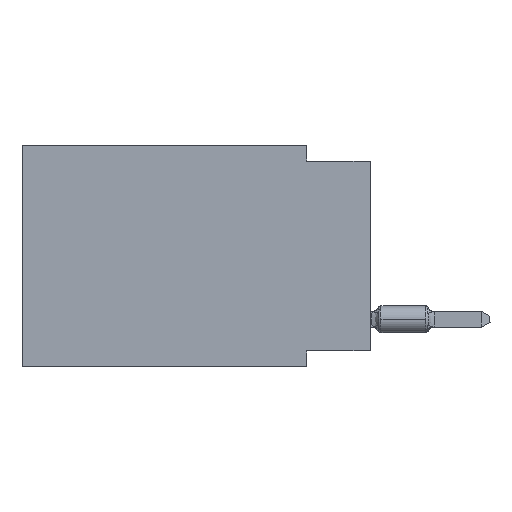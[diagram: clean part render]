
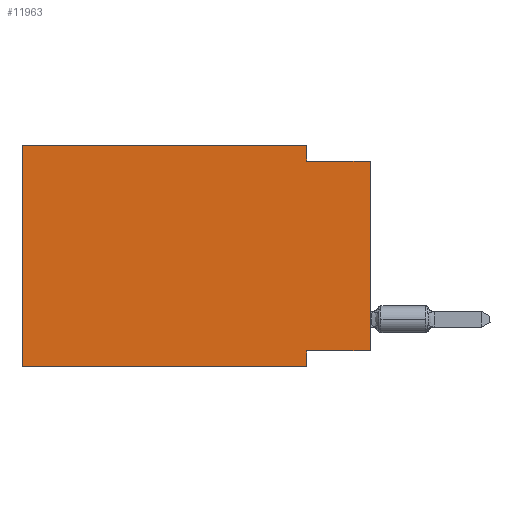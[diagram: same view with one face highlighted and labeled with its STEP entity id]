
A CAD part, left-side view. The second image highlights one B-rep face of the part: STEP entity #11963.
In plain terms, the highlighted planar face has unit normal (-1, 0, 0).
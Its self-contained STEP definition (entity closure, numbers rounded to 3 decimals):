
#720 = VERTEX_POINT ( 'NONE', #41587 ) ;
#2202 = DIRECTION ( 'NONE',  ( 1., 0., 0. ) ) ;
#2887 = ORIENTED_EDGE ( 'NONE', *, *, #34337, .F. ) ;
#4455 = EDGE_CURVE ( 'NONE', #20616, #720, #30341, .T. ) ;
#5521 = VECTOR ( 'NONE', #42073, 1000. ) ;
#6248 = VERTEX_POINT ( 'NONE', #16969 ) ;
#6534 = ORIENTED_EDGE ( 'NONE', *, *, #30725, .F. ) ;
#6631 = VECTOR ( 'NONE', #8242, 1000. ) ;
#7049 = LINE ( 'NONE', #21223, #22785 ) ;
#7694 = EDGE_LOOP ( 'NONE', ( #36475, #6534, #2887, #10210, #45464, #29347, #35352, #25045 ) ) ;
#7738 = CARTESIAN_POINT ( 'NONE',  ( 0., 0., -8.255 ) ) ;
#8242 = DIRECTION ( 'NONE',  ( 0., -1., 0. ) ) ;
#8976 = CARTESIAN_POINT ( 'NONE',  ( 0., 13.97, 0. ) ) ;
#10210 = ORIENTED_EDGE ( 'NONE', *, *, #4455, .F. ) ;
#10689 = VERTEX_POINT ( 'NONE', #41437 ) ;
#11297 = CARTESIAN_POINT ( 'NONE',  ( 0., 0., -0.635 ) ) ;
#11431 = DIRECTION ( 'NONE',  ( 0., 0., 1. ) ) ;
#11503 = LINE ( 'NONE', #19587, #6631 ) ;
#11963 = ADVANCED_FACE ( 'NONE', ( #30326 ), #44464, .F. ) ;
#12104 = CARTESIAN_POINT ( 'NONE',  ( 0., 2.54, -8.89 ) ) ;
#12562 = DIRECTION ( 'NONE',  ( 0., 0., -1. ) ) ;
#13412 = VECTOR ( 'NONE', #33971, 1000. ) ;
#13740 = VECTOR ( 'NONE', #12562, 1000. ) ;
#13763 = LINE ( 'NONE', #41613, #5521 ) ;
#15521 = VECTOR ( 'NONE', #20331, 1000. ) ;
#15610 = CARTESIAN_POINT ( 'NONE',  ( 0., 0., 0. ) ) ;
#15676 = EDGE_CURVE ( 'NONE', #17171, #20616, #43720, .T. ) ;
#16839 = CARTESIAN_POINT ( 'NONE',  ( 0., 13.97, 0. ) ) ;
#16969 = CARTESIAN_POINT ( 'NONE',  ( 0., 2.54, -8.89 ) ) ;
#17171 = VERTEX_POINT ( 'NONE', #43121 ) ;
#17316 = CARTESIAN_POINT ( 'NONE',  ( 0., 2.54, -0.635 ) ) ;
#19587 = CARTESIAN_POINT ( 'NONE',  ( 0., 13.97, -8.89 ) ) ;
#19666 = CARTESIAN_POINT ( 'NONE',  ( 0., 0., -8.255 ) ) ;
#20331 = DIRECTION ( 'NONE',  ( 0., -1., 0. ) ) ;
#20616 = VERTEX_POINT ( 'NONE', #43680 ) ;
#21223 = CARTESIAN_POINT ( 'NONE',  ( 0., 0., -0.635 ) ) ;
#22308 = EDGE_CURVE ( 'NONE', #22930, #10689, #22350, .T. ) ;
#22350 = LINE ( 'NONE', #7738, #42764 ) ;
#22785 = VECTOR ( 'NONE', #38169, 1000. ) ;
#22930 = VERTEX_POINT ( 'NONE', #19666 ) ;
#23051 = CARTESIAN_POINT ( 'NONE',  ( 0., 13.97, 0. ) ) ;
#25045 = ORIENTED_EDGE ( 'NONE', *, *, #22308, .F. ) ;
#28871 = DIRECTION ( 'NONE',  ( 0., 1., 0. ) ) ;
#29347 = ORIENTED_EDGE ( 'NONE', *, *, #39469, .T. ) ;
#29542 = LINE ( 'NONE', #12104, #13740 ) ;
#30326 = FACE_OUTER_BOUND ( 'NONE', #7694, .T. ) ;
#30341 = LINE ( 'NONE', #8976, #15521 ) ;
#30725 = EDGE_CURVE ( 'NONE', #38875, #33691, #7049, .T. ) ;
#31015 = DIRECTION ( 'NONE',  ( 0., 0., -1. ) ) ;
#31702 = AXIS2_PLACEMENT_3D ( 'NONE', #16839, #2202, #31015 ) ;
#33691 = VERTEX_POINT ( 'NONE', #11297 ) ;
#33971 = DIRECTION ( 'NONE',  ( 0., 0., 1. ) ) ;
#34337 = EDGE_CURVE ( 'NONE', #720, #38875, #13763, .T. ) ;
#34655 = EDGE_CURVE ( 'NONE', #10689, #6248, #29542, .T. ) ;
#35352 = ORIENTED_EDGE ( 'NONE', *, *, #34655, .F. ) ;
#35438 = EDGE_CURVE ( 'NONE', #22930, #33691, #43681, .T. ) ;
#36475 = ORIENTED_EDGE ( 'NONE', *, *, #35438, .T. ) ;
#36846 = VECTOR ( 'NONE', #11431, 1000. ) ;
#38169 = DIRECTION ( 'NONE',  ( 0., -1., 0. ) ) ;
#38875 = VERTEX_POINT ( 'NONE', #17316 ) ;
#39469 = EDGE_CURVE ( 'NONE', #17171, #6248, #11503, .T. ) ;
#41437 = CARTESIAN_POINT ( 'NONE',  ( 0., 2.54, -8.255 ) ) ;
#41587 = CARTESIAN_POINT ( 'NONE',  ( 0., 2.54, 0. ) ) ;
#41613 = CARTESIAN_POINT ( 'NONE',  ( 0., 2.54, 0. ) ) ;
#42073 = DIRECTION ( 'NONE',  ( 0., 0., -1. ) ) ;
#42764 = VECTOR ( 'NONE', #28871, 1000. ) ;
#43121 = CARTESIAN_POINT ( 'NONE',  ( 0., 13.97, -8.89 ) ) ;
#43680 = CARTESIAN_POINT ( 'NONE',  ( 0., 13.97, 0. ) ) ;
#43681 = LINE ( 'NONE', #15610, #36846 ) ;
#43720 = LINE ( 'NONE', #23051, #13412 ) ;
#44464 = PLANE ( 'NONE',  #31702 ) ;
#45464 = ORIENTED_EDGE ( 'NONE', *, *, #15676, .F. ) ;
